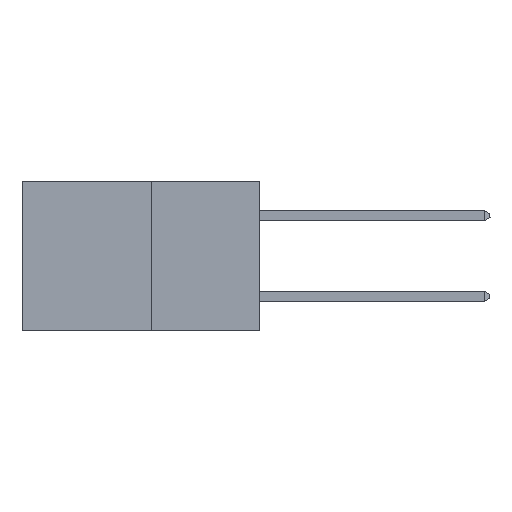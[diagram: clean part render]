
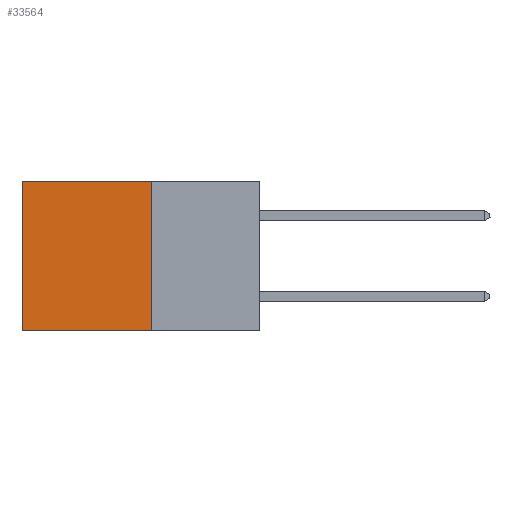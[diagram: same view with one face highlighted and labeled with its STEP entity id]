
A CAD part, left-side view. The second image highlights one B-rep face of the part: STEP entity #33564.
In plain terms, the highlighted planar face has unit normal (-1, 0, 0).
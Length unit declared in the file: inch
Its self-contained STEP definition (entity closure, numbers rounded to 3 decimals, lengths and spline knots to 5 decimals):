
#343 = DIRECTION ( 'NONE',  ( 0., 0., -1. ) ) ;
#2774 = CARTESIAN_POINT ( 'NONE',  ( 0.277, 0.27, -0.37 ) ) ;
#2900 = LINE ( 'NONE', #18343, #31067 ) ;
#3179 = LINE ( 'NONE', #23178, #24143 ) ;
#3693 = VERTEX_POINT ( 'NONE', #17634 ) ;
#4534 = LINE ( 'NONE', #2774, #25447 ) ;
#7252 = EDGE_CURVE ( 'NONE', #24159, #3693, #3179, .T. ) ;
#8598 = DIRECTION ( 'NONE',  ( 0., 1., 0. ) ) ;
#8623 = EDGE_LOOP ( 'NONE', ( #22297, #33525, #8967, #22770 ) ) ;
#8967 = ORIENTED_EDGE ( 'NONE', *, *, #26500, .F. ) ;
#14622 = CARTESIAN_POINT ( 'NONE',  ( 0.277, 0.27, -0.37 ) ) ;
#14776 = AXIS2_PLACEMENT_3D ( 'NONE', #22180, #16823, #343 ) ;
#15017 = VERTEX_POINT ( 'NONE', #22647 ) ;
#15071 = DIRECTION ( 'NONE',  ( 0., 1., 0. ) ) ;
#16463 = DIRECTION ( 'NONE',  ( 0., 0., -1. ) ) ;
#16823 = DIRECTION ( 'NONE',  ( 1., 0., 0. ) ) ;
#17634 = CARTESIAN_POINT ( 'NONE',  ( 0.277, 0.59, 0. ) ) ;
#17796 = FACE_OUTER_BOUND ( 'NONE', #8623, .T. ) ;
#18343 = CARTESIAN_POINT ( 'NONE',  ( 0.277, 0.59, -0.37 ) ) ;
#19396 = EDGE_CURVE ( 'NONE', #34653, #15017, #31793, .T. ) ;
#22180 = CARTESIAN_POINT ( 'NONE',  ( 0.277, 0.27, -0.37 ) ) ;
#22238 = CARTESIAN_POINT ( 'NONE',  ( 0.277, 0.27, -0.37 ) ) ;
#22297 = ORIENTED_EDGE ( 'NONE', *, *, #32006, .T. ) ;
#22647 = CARTESIAN_POINT ( 'NONE',  ( 0.277, 0.59, -0.37 ) ) ;
#22770 = ORIENTED_EDGE ( 'NONE', *, *, #7252, .T. ) ;
#23178 = CARTESIAN_POINT ( 'NONE',  ( 0.277, 0.27, 0. ) ) ;
#24143 = VECTOR ( 'NONE', #15071, 39.37008 ) ;
#24159 = VERTEX_POINT ( 'NONE', #31123 ) ;
#25447 = VECTOR ( 'NONE', #16463, 39.37008 ) ;
#26500 = EDGE_CURVE ( 'NONE', #24159, #34653, #4534, .T. ) ;
#27617 = PLANE ( 'NONE',  #14776 ) ;
#30955 = VECTOR ( 'NONE', #8598, 39.37008 ) ;
#31067 = VECTOR ( 'NONE', #31841, 39.37008 ) ;
#31123 = CARTESIAN_POINT ( 'NONE',  ( 0.277, 0.27, 0. ) ) ;
#31793 = LINE ( 'NONE', #22238, #30955 ) ;
#31841 = DIRECTION ( 'NONE',  ( 0., 0., -1. ) ) ;
#32006 = EDGE_CURVE ( 'NONE', #3693, #15017, #2900, .T. ) ;
#33525 = ORIENTED_EDGE ( 'NONE', *, *, #19396, .F. ) ;
#33564 = ADVANCED_FACE ( 'NONE', ( #17796 ), #27617, .F. ) ;
#34653 = VERTEX_POINT ( 'NONE', #14622 ) ;
